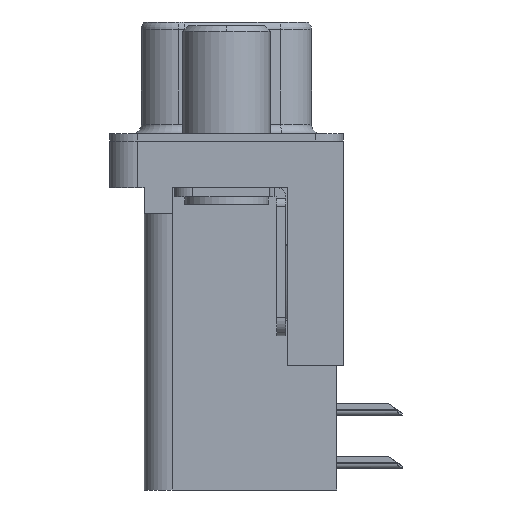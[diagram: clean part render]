
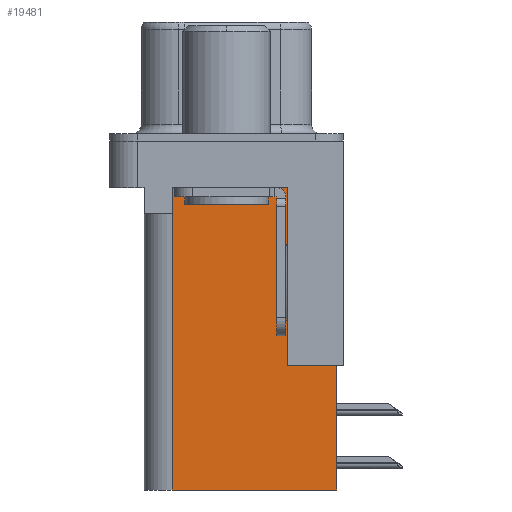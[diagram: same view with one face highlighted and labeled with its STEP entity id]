
A CAD part, left-side view. The second image highlights one B-rep face of the part: STEP entity #19481.
In plain terms, the highlighted planar face has unit normal (-1, 0, 0).
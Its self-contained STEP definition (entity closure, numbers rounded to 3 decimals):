
#866 = VECTOR ( 'NONE', #19032, 1000. ) ;
#1364 = VECTOR ( 'NONE', #11707, 1000. ) ;
#1516 = ORIENTED_EDGE ( 'NONE', *, *, #20730, .T. ) ;
#1911 = LINE ( 'NONE', #7058, #10767 ) ;
#1957 = CARTESIAN_POINT ( 'NONE',  ( 3.7, -5.925, -2. ) ) ;
#2020 = ORIENTED_EDGE ( 'NONE', *, *, #11259, .T. ) ;
#2241 = DIRECTION ( 'NONE',  ( 0., 1., 0. ) ) ;
#3405 = CARTESIAN_POINT ( 'NONE',  ( 3.7, 2.925, -3.9 ) ) ;
#3417 = VECTOR ( 'NONE', #8338, 1000. ) ;
#3651 = CARTESIAN_POINT ( 'NONE',  ( 3.7, 0., -3.9 ) ) ;
#4000 = VECTOR ( 'NONE', #2241, 1000. ) ;
#4018 = LINE ( 'NONE', #21276, #9020 ) ;
#4180 = CARTESIAN_POINT ( 'NONE',  ( 3.7, 2.925, -18.76 ) ) ;
#4438 = VECTOR ( 'NONE', #9327, 1000. ) ;
#4621 = CARTESIAN_POINT ( 'NONE',  ( 3.7, 2.895, -2.5 ) ) ;
#6376 = FACE_OUTER_BOUND ( 'NONE', #8815, .T. ) ;
#6498 = DIRECTION ( 'NONE',  ( 0., 1., 0. ) ) ;
#7058 = CARTESIAN_POINT ( 'NONE',  ( 3.7, -6.295, -12.05 ) ) ;
#7248 = CARTESIAN_POINT ( 'NONE',  ( 3.7, -5.925, -18.76 ) ) ;
#7361 = EDGE_CURVE ( 'NONE', #14145, #8109, #7778, .T. ) ;
#7422 = VERTEX_POINT ( 'NONE', #8023 ) ;
#7778 = LINE ( 'NONE', #13605, #4000 ) ;
#8023 = CARTESIAN_POINT ( 'NONE',  ( 3.7, -3.295, -12.05 ) ) ;
#8109 = VERTEX_POINT ( 'NONE', #10664 ) ;
#8142 = ORIENTED_EDGE ( 'NONE', *, *, #7361, .F. ) ;
#8338 = DIRECTION ( 'NONE',  ( 0., 0., 1. ) ) ;
#8724 = ORIENTED_EDGE ( 'NONE', *, *, #11262, .T. ) ;
#8815 = EDGE_LOOP ( 'NONE', ( #8724, #22293, #2020, #13314, #8142, #18287, #11642, #1516 ) ) ;
#8954 = VERTEX_POINT ( 'NONE', #24365 ) ;
#9020 = VECTOR ( 'NONE', #17421, 1000. ) ;
#9327 = DIRECTION ( 'NONE',  ( 0., 1., 0. ) ) ;
#9347 = CARTESIAN_POINT ( 'NONE',  ( 3.7, -3.295, -2.5 ) ) ;
#10664 = CARTESIAN_POINT ( 'NONE',  ( 3.7, 2.925, -18.76 ) ) ;
#10767 = VECTOR ( 'NONE', #16632, 1000. ) ;
#11258 = DIRECTION ( 'NONE',  ( 0., 1., 0. ) ) ;
#11259 = EDGE_CURVE ( 'NONE', #8954, #19723, #24187, .T. ) ;
#11262 = EDGE_CURVE ( 'NONE', #22034, #19517, #23575, .T. ) ;
#11394 = LINE ( 'NONE', #4180, #1364 ) ;
#11642 = ORIENTED_EDGE ( 'NONE', *, *, #24565, .T. ) ;
#11707 = DIRECTION ( 'NONE',  ( 0., 0., 1. ) ) ;
#12538 = EDGE_CURVE ( 'NONE', #18726, #14145, #21747, .T. ) ;
#13314 = ORIENTED_EDGE ( 'NONE', *, *, #20589, .F. ) ;
#13605 = CARTESIAN_POINT ( 'NONE',  ( 3.7, -3.295, -18.76 ) ) ;
#14101 = LINE ( 'NONE', #19871, #3417 ) ;
#14112 = PLANE ( 'NONE',  #23128 ) ;
#14145 = VERTEX_POINT ( 'NONE', #7248 ) ;
#16030 = CARTESIAN_POINT ( 'NONE',  ( 3.7, -3.295, -18.76 ) ) ;
#16632 = DIRECTION ( 'NONE',  ( 0., 1., 0. ) ) ;
#17421 = DIRECTION ( 'NONE',  ( 0., 0., -1. ) ) ;
#17977 = DIRECTION ( 'NONE',  ( 1., 0., 0. ) ) ;
#18287 = ORIENTED_EDGE ( 'NONE', *, *, #12538, .F. ) ;
#18502 = VECTOR ( 'NONE', #11258, 1000. ) ;
#18726 = VERTEX_POINT ( 'NONE', #23707 ) ;
#19032 = DIRECTION ( 'NONE',  ( 0., 0., -1. ) ) ;
#19481 = ADVANCED_FACE ( 'NONE', ( #6376 ), #14112, .F. ) ;
#19517 = VERTEX_POINT ( 'NONE', #4621 ) ;
#19723 = VERTEX_POINT ( 'NONE', #3405 ) ;
#19871 = CARTESIAN_POINT ( 'NONE',  ( 3.7, -3.295, -18.76 ) ) ;
#20589 = EDGE_CURVE ( 'NONE', #8109, #19723, #11394, .T. ) ;
#20730 = EDGE_CURVE ( 'NONE', #7422, #22034, #14101, .T. ) ;
#21276 = CARTESIAN_POINT ( 'NONE',  ( 3.7, 2.895, -3.9 ) ) ;
#21747 = LINE ( 'NONE', #1957, #866 ) ;
#22034 = VERTEX_POINT ( 'NONE', #9347 ) ;
#22130 = EDGE_CURVE ( 'NONE', #19517, #8954, #4018, .T. ) ;
#22293 = ORIENTED_EDGE ( 'NONE', *, *, #22130, .T. ) ;
#22774 = CARTESIAN_POINT ( 'NONE',  ( 3.7, -3.295, -2.5 ) ) ;
#23128 = AXIS2_PLACEMENT_3D ( 'NONE', #16030, #17977, #6498 ) ;
#23575 = LINE ( 'NONE', #22774, #4438 ) ;
#23707 = CARTESIAN_POINT ( 'NONE',  ( 3.7, -5.925, -12.05 ) ) ;
#24187 = LINE ( 'NONE', #3651, #18502 ) ;
#24365 = CARTESIAN_POINT ( 'NONE',  ( 3.7, 2.895, -3.9 ) ) ;
#24565 = EDGE_CURVE ( 'NONE', #18726, #7422, #1911, .T. ) ;
